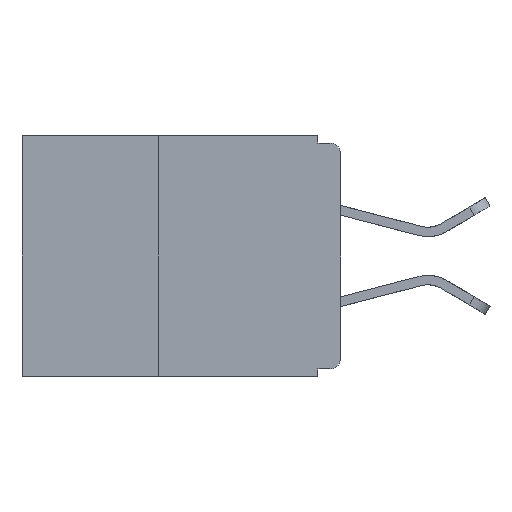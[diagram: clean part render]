
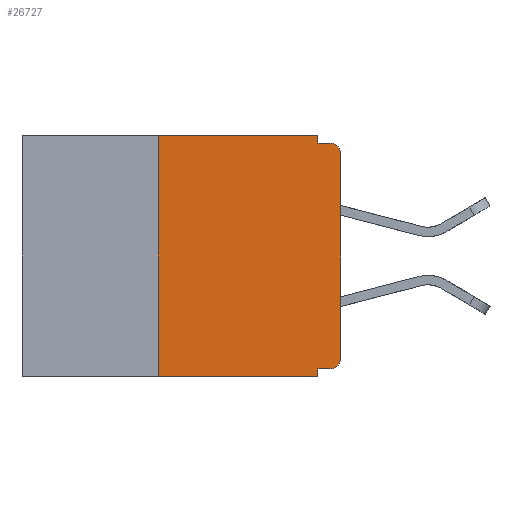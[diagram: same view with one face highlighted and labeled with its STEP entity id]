
A CAD part, left-side view. The second image highlights one B-rep face of the part: STEP entity #26727.
In plain terms, the highlighted planar face has unit normal (-1, 0, 0).
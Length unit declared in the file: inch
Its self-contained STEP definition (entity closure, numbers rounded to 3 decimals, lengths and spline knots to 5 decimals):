
#393 = LINE ( 'NONE', #31478, #16576 ) ;
#512 = DIRECTION ( 'NONE',  ( 0., 0., 1. ) ) ;
#945 = EDGE_CURVE ( 'NONE', #1488, #31870, #393, .T. ) ;
#1014 = DIRECTION ( 'NONE',  ( 0., 0., -1. ) ) ;
#1048 = VERTEX_POINT ( 'NONE', #28270 ) ;
#1488 = VERTEX_POINT ( 'NONE', #12676 ) ;
#1496 = EDGE_CURVE ( 'NONE', #19829, #10903, #20486, .T. ) ;
#2336 = DIRECTION ( 'NONE',  ( 0., 0., -1. ) ) ;
#2615 = VECTOR ( 'NONE', #27800, 39.37008 ) ;
#2752 = EDGE_CURVE ( 'NONE', #15571, #18868, #32021, .T. ) ;
#2807 = CARTESIAN_POINT ( 'NONE',  ( 0., 0., -0.01 ) ) ;
#3284 = ORIENTED_EDGE ( 'NONE', *, *, #16830, .T. ) ;
#4158 = VERTEX_POINT ( 'NONE', #11211 ) ;
#4159 = ORIENTED_EDGE ( 'NONE', *, *, #20053, .F. ) ;
#4281 = PLANE ( 'NONE',  #5898 ) ;
#4290 = ORIENTED_EDGE ( 'NONE', *, *, #20041, .F. ) ;
#4602 = CARTESIAN_POINT ( 'NONE',  ( 0., 0.015, -0.32 ) ) ;
#4913 = VECTOR ( 'NONE', #22579, 39.37008 ) ;
#5798 = ORIENTED_EDGE ( 'NONE', *, *, #2752, .F. ) ;
#5898 = AXIS2_PLACEMENT_3D ( 'NONE', #29503, #7001, #24088 ) ;
#5988 = LINE ( 'NONE', #14840, #34910 ) ;
#7001 = DIRECTION ( 'NONE',  ( 1., 0., 0. ) ) ;
#7204 = VERTEX_POINT ( 'NONE', #4602 ) ;
#7320 = ORIENTED_EDGE ( 'NONE', *, *, #25341, .F. ) ;
#9692 = VECTOR ( 'NONE', #35336, 39.37008 ) ;
#10005 = VERTEX_POINT ( 'NONE', #30359 ) ;
#10086 = ORIENTED_EDGE ( 'NONE', *, *, #13855, .T. ) ;
#10446 = ORIENTED_EDGE ( 'NONE', *, *, #27574, .F. ) ;
#10741 = ORIENTED_EDGE ( 'NONE', *, *, #945, .T. ) ;
#10903 = VERTEX_POINT ( 'NONE', #28745 ) ;
#11211 = CARTESIAN_POINT ( 'NONE',  ( 0., 0.015, -0.01 ) ) ;
#11714 = FACE_OUTER_BOUND ( 'NONE', #31111, .T. ) ;
#12056 = DIRECTION ( 'NONE',  ( 0., 1., 0. ) ) ;
#12382 = DIRECTION ( 'NONE',  ( 0., 0., -1. ) ) ;
#12676 = CARTESIAN_POINT ( 'NONE',  ( 0., 0., -0.305 ) ) ;
#12745 = VECTOR ( 'NONE', #12056, 39.37008 ) ;
#13013 = CARTESIAN_POINT ( 'NONE',  ( 0., 0.031, -0.33 ) ) ;
#13855 = EDGE_CURVE ( 'NONE', #7204, #1488, #22052, .T. ) ;
#14840 = CARTESIAN_POINT ( 'NONE',  ( 0., 0.25, -0.33 ) ) ;
#14961 = ORIENTED_EDGE ( 'NONE', *, *, #34886, .T. ) ;
#15434 = CARTESIAN_POINT ( 'NONE',  ( 0., 0.031, -0.32 ) ) ;
#15571 = VERTEX_POINT ( 'NONE', #27396 ) ;
#16576 = VECTOR ( 'NONE', #31563, 39.37008 ) ;
#16830 = EDGE_CURVE ( 'NONE', #10005, #10903, #18757, .T. ) ;
#17110 = DIRECTION ( 'NONE',  ( 0., -1., 0. ) ) ;
#17740 = ORIENTED_EDGE ( 'NONE', *, *, #1496, .F. ) ;
#18203 = DIRECTION ( 'NONE',  ( -1., 0., 0. ) ) ;
#18757 = LINE ( 'NONE', #19626, #2615 ) ;
#18868 = VERTEX_POINT ( 'NONE', #36107 ) ;
#19475 = DIRECTION ( 'NONE',  ( -1., 0., 0. ) ) ;
#19626 = CARTESIAN_POINT ( 'NONE',  ( 0., 0.437, -0.33 ) ) ;
#19829 = VERTEX_POINT ( 'NONE', #15434 ) ;
#20041 = EDGE_CURVE ( 'NONE', #10005, #1048, #5988, .T. ) ;
#20053 = EDGE_CURVE ( 'NONE', #7204, #19829, #22005, .T. ) ;
#20486 = LINE ( 'NONE', #13013, #26948 ) ;
#22005 = LINE ( 'NONE', #34322, #12745 ) ;
#22015 = AXIS2_PLACEMENT_3D ( 'NONE', #34674, #18203, #1014 ) ;
#22052 = CIRCLE ( 'NONE', #22015, 0.015 ) ;
#22579 = DIRECTION ( 'NONE',  ( 0., -1., 0. ) ) ;
#24088 = DIRECTION ( 'NONE',  ( 0., 0., -1. ) ) ;
#24449 = CIRCLE ( 'NONE', #28985, 0.015 ) ;
#25341 = EDGE_CURVE ( 'NONE', #18868, #4158, #27972, .T. ) ;
#26727 = ADVANCED_FACE ( 'NONE', ( #11714 ), #4281, .F. ) ;
#26948 = VECTOR ( 'NONE', #12382, 39.37008 ) ;
#27113 = VECTOR ( 'NONE', #17110, 39.37008 ) ;
#27396 = CARTESIAN_POINT ( 'NONE',  ( 0., 0.031, 0. ) ) ;
#27426 = LINE ( 'NONE', #33537, #4913 ) ;
#27574 = EDGE_CURVE ( 'NONE', #1048, #15571, #27426, .T. ) ;
#27800 = DIRECTION ( 'NONE',  ( 0., -1., 0. ) ) ;
#27972 = LINE ( 'NONE', #2807, #27113 ) ;
#28270 = CARTESIAN_POINT ( 'NONE',  ( 0., 0.25, 0. ) ) ;
#28745 = CARTESIAN_POINT ( 'NONE',  ( 0., 0.031, -0.33 ) ) ;
#28985 = AXIS2_PLACEMENT_3D ( 'NONE', #35890, #19475, #2336 ) ;
#29503 = CARTESIAN_POINT ( 'NONE',  ( 0., 0.437, 0. ) ) ;
#30359 = CARTESIAN_POINT ( 'NONE',  ( 0., 0.25, -0.33 ) ) ;
#31111 = EDGE_LOOP ( 'NONE', ( #10741, #14961, #7320, #5798, #10446, #4290, #3284, #17740, #4159, #10086 ) ) ;
#31478 = CARTESIAN_POINT ( 'NONE',  ( 0., 0., 0. ) ) ;
#31563 = DIRECTION ( 'NONE',  ( 0., 0., 1. ) ) ;
#31870 = VERTEX_POINT ( 'NONE', #32982 ) ;
#32021 = LINE ( 'NONE', #34830, #9692 ) ;
#32982 = CARTESIAN_POINT ( 'NONE',  ( 0., 0., -0.025 ) ) ;
#33537 = CARTESIAN_POINT ( 'NONE',  ( 0., 0.437, 0. ) ) ;
#34322 = CARTESIAN_POINT ( 'NONE',  ( 0., 0., -0.32 ) ) ;
#34674 = CARTESIAN_POINT ( 'NONE',  ( 0., 0.015, -0.305 ) ) ;
#34830 = CARTESIAN_POINT ( 'NONE',  ( 0., 0.031, 0. ) ) ;
#34886 = EDGE_CURVE ( 'NONE', #31870, #4158, #24449, .T. ) ;
#34910 = VECTOR ( 'NONE', #512, 39.37008 ) ;
#35336 = DIRECTION ( 'NONE',  ( 0., 0., -1. ) ) ;
#35890 = CARTESIAN_POINT ( 'NONE',  ( 0., 0.015, -0.025 ) ) ;
#36107 = CARTESIAN_POINT ( 'NONE',  ( 0., 0.031, -0.01 ) ) ;
